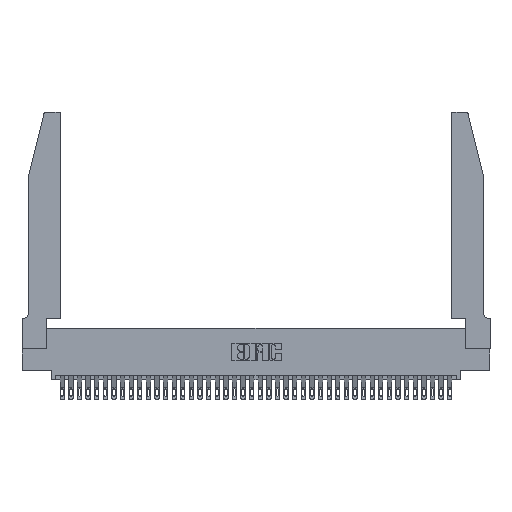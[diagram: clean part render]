
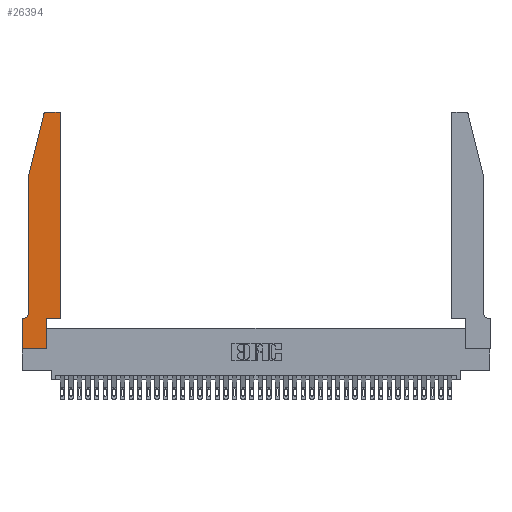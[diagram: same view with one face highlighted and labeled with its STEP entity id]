
A CAD part, top view. The second image highlights one B-rep face of the part: STEP entity #26394.
In plain terms, the highlighted planar face has unit normal (0, 0, 1).
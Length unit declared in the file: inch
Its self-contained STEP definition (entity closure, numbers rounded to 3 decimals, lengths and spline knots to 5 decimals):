
#623 = CARTESIAN_POINT ( 'NONE',  ( 0.4505, 0.35, 0.37 ) ) ;
#1113 = EDGE_CURVE ( 'NONE', #15938, #35383, #37531, .T. ) ;
#1392 = EDGE_CURVE ( 'NONE', #5503, #29788, #25211, .T. ) ;
#1678 = VERTEX_POINT ( 'NONE', #5254 ) ;
#1770 = EDGE_CURVE ( 'NONE', #29566, #25575, #26668, .T. ) ;
#1964 = CARTESIAN_POINT ( 'NONE',  ( 0.4505, 2.72, 0.37 ) ) ;
#2930 = FACE_OUTER_BOUND ( 'NONE', #30927, .T. ) ;
#2972 = EDGE_CURVE ( 'NONE', #29788, #29566, #28120, .T. ) ;
#3260 = VECTOR ( 'NONE', #28836, 39.37008 ) ;
#4266 = LINE ( 'NONE', #39532, #8136 ) ;
#4419 = VECTOR ( 'NONE', #25385, 39.37008 ) ;
#4619 = VECTOR ( 'NONE', #27135, 39.37008 ) ;
#4669 = ORIENTED_EDGE ( 'NONE', *, *, #36475, .T. ) ;
#4964 = CIRCLE ( 'NONE', #12830, 0.03 ) ;
#5254 = CARTESIAN_POINT ( 'NONE',  ( 0.4505, 0.35, 0.37 ) ) ;
#5293 = ORIENTED_EDGE ( 'NONE', *, *, #1392, .T. ) ;
#5503 = VERTEX_POINT ( 'NONE', #6472 ) ;
#6472 = CARTESIAN_POINT ( 'NONE',  ( 0.0755, 0.42, 0.37 ) ) ;
#6616 = DIRECTION ( 'NONE',  ( -1., 0., 0. ) ) ;
#7291 = CARTESIAN_POINT ( 'NONE',  ( 0.2865, 0., 0.37 ) ) ;
#7638 = LINE ( 'NONE', #13547, #30873 ) ;
#7755 = VERTEX_POINT ( 'NONE', #27853 ) ;
#7964 = CARTESIAN_POINT ( 'NONE',  ( 0.2865, 0.35, 0.37 ) ) ;
#8090 = DIRECTION ( 'NONE',  ( 1., 0., 0. ) ) ;
#8136 = VECTOR ( 'NONE', #36692, 39.37008 ) ;
#8575 = CARTESIAN_POINT ( 'NONE',  ( 0.284, 2.72, 0.37 ) ) ;
#8647 = DIRECTION ( 'NONE',  ( 0., -1., 0. ) ) ;
#8649 = ORIENTED_EDGE ( 'NONE', *, *, #12506, .T. ) ;
#8650 = CARTESIAN_POINT ( 'NONE',  ( 0., 0., 0.37 ) ) ;
#9004 = EDGE_CURVE ( 'NONE', #18876, #24777, #7638, .T. ) ;
#9060 = EDGE_CURVE ( 'NONE', #1678, #15938, #4266, .T. ) ;
#9557 = LINE ( 'NONE', #29116, #27879 ) ;
#9665 = DIRECTION ( 'NONE',  ( 0., 0., -1. ) ) ;
#10341 = ORIENTED_EDGE ( 'NONE', *, *, #37391, .T. ) ;
#10510 = ORIENTED_EDGE ( 'NONE', *, *, #31193, .T. ) ;
#10764 = CARTESIAN_POINT ( 'NONE',  ( 0., 0.35, 0.37 ) ) ;
#11015 = ORIENTED_EDGE ( 'NONE', *, *, #1770, .T. ) ;
#12506 = EDGE_CURVE ( 'NONE', #13394, #13069, #24665, .T. ) ;
#12652 = ORIENTED_EDGE ( 'NONE', *, *, #9004, .T. ) ;
#12830 = AXIS2_PLACEMENT_3D ( 'NONE', #8575, #24651, #21610 ) ;
#13069 = VERTEX_POINT ( 'NONE', #33741 ) ;
#13394 = VERTEX_POINT ( 'NONE', #38401 ) ;
#13547 = CARTESIAN_POINT ( 'NONE',  ( 0.2865, 0.35, 0.37 ) ) ;
#14224 = DIRECTION ( 'NONE',  ( -1., 0., 0. ) ) ;
#15938 = VERTEX_POINT ( 'NONE', #1964 ) ;
#17227 = DIRECTION ( 'NONE',  ( 1., 0., 0. ) ) ;
#17337 = CARTESIAN_POINT ( 'NONE',  ( 0.4205, 2.72, 0.37 ) ) ;
#18331 = ORIENTED_EDGE ( 'NONE', *, *, #2972, .T. ) ;
#18876 = VERTEX_POINT ( 'NONE', #7291 ) ;
#19086 = CARTESIAN_POINT ( 'NONE',  ( 0.0055, 0.42, 0.37 ) ) ;
#19629 = EDGE_CURVE ( 'NONE', #7755, #13394, #4964, .T. ) ;
#21147 = VECTOR ( 'NONE', #14224, 39.37008 ) ;
#21576 = DIRECTION ( 'NONE',  ( 0., -1., 0. ) ) ;
#21610 = DIRECTION ( 'NONE',  ( 1., 0., 0. ) ) ;
#22152 = CARTESIAN_POINT ( 'NONE',  ( 0.0055, 0.35, 0.37 ) ) ;
#22228 = VECTOR ( 'NONE', #8647, 39.37008 ) ;
#22506 = LINE ( 'NONE', #623, #3260 ) ;
#23856 = ORIENTED_EDGE ( 'NONE', *, *, #31564, .T. ) ;
#24651 = DIRECTION ( 'NONE',  ( 0., 0., 1. ) ) ;
#24665 = LINE ( 'NONE', #29022, #4419 ) ;
#24777 = VERTEX_POINT ( 'NONE', #7964 ) ;
#25211 = CIRCLE ( 'NONE', #33574, 0.07 ) ;
#25385 = DIRECTION ( 'NONE',  ( -0.239, -0.971, 0. ) ) ;
#25575 = VERTEX_POINT ( 'NONE', #8650 ) ;
#25917 = DIRECTION ( 'NONE',  ( 1., 0., 0. ) ) ;
#26025 = CARTESIAN_POINT ( 'NONE',  ( 0.0755, 0.35, 0.37 ) ) ;
#26394 = ADVANCED_FACE ( 'NONE', ( #2930 ), #32864, .T. ) ;
#26618 = AXIS2_PLACEMENT_3D ( 'NONE', #17337, #27053, #8090 ) ;
#26668 = LINE ( 'NONE', #27338, #22228 ) ;
#26930 = CARTESIAN_POINT ( 'NONE',  ( 0., 0.35, 0.37 ) ) ;
#27053 = DIRECTION ( 'NONE',  ( 0., 0., 1. ) ) ;
#27135 = DIRECTION ( 'NONE',  ( -1., 0., 0. ) ) ;
#27338 = CARTESIAN_POINT ( 'NONE',  ( 0., 0., 0.37 ) ) ;
#27853 = CARTESIAN_POINT ( 'NONE',  ( 0.284, 2.75, 0.37 ) ) ;
#27879 = VECTOR ( 'NONE', #25917, 39.37008 ) ;
#28120 = LINE ( 'NONE', #26025, #21147 ) ;
#28436 = VECTOR ( 'NONE', #21576, 39.37008 ) ;
#28836 = DIRECTION ( 'NONE',  ( 1., 0., 0. ) ) ;
#28933 = LINE ( 'NONE', #34242, #28436 ) ;
#29022 = CARTESIAN_POINT ( 'NONE',  ( 0.0755, 2., 0.37 ) ) ;
#29116 = CARTESIAN_POINT ( 'NONE',  ( 0., 0., 0.37 ) ) ;
#29490 = CARTESIAN_POINT ( 'NONE',  ( 0.4205, 2.75, 0.37 ) ) ;
#29566 = VERTEX_POINT ( 'NONE', #10764 ) ;
#29788 = VERTEX_POINT ( 'NONE', #22152 ) ;
#30873 = VECTOR ( 'NONE', #30973, 39.37008 ) ;
#30927 = EDGE_LOOP ( 'NONE', ( #23856, #32319, #8649, #10341, #5293, #18331, #11015, #10510, #12652, #4669, #37583, #39095 ) ) ;
#30973 = DIRECTION ( 'NONE',  ( 0., 1., 0. ) ) ;
#31193 = EDGE_CURVE ( 'NONE', #25575, #18876, #9557, .T. ) ;
#31564 = EDGE_CURVE ( 'NONE', #35383, #7755, #36206, .T. ) ;
#32319 = ORIENTED_EDGE ( 'NONE', *, *, #19629, .T. ) ;
#32864 = PLANE ( 'NONE',  #40697 ) ;
#33574 = AXIS2_PLACEMENT_3D ( 'NONE', #19086, #9665, #6616 ) ;
#33741 = CARTESIAN_POINT ( 'NONE',  ( 0.0755, 2., 0.37 ) ) ;
#34242 = CARTESIAN_POINT ( 'NONE',  ( 0.0755, 2., 0.37 ) ) ;
#35383 = VERTEX_POINT ( 'NONE', #29490 ) ;
#36168 = DIRECTION ( 'NONE',  ( 0., 0., 1. ) ) ;
#36206 = LINE ( 'NONE', #39599, #4619 ) ;
#36475 = EDGE_CURVE ( 'NONE', #24777, #1678, #22506, .T. ) ;
#36692 = DIRECTION ( 'NONE',  ( 0., 1., 0. ) ) ;
#37391 = EDGE_CURVE ( 'NONE', #13069, #5503, #28933, .T. ) ;
#37531 = CIRCLE ( 'NONE', #26618, 0.03 ) ;
#37583 = ORIENTED_EDGE ( 'NONE', *, *, #9060, .T. ) ;
#38401 = CARTESIAN_POINT ( 'NONE',  ( 0.25487, 2.72718, 0.37 ) ) ;
#39095 = ORIENTED_EDGE ( 'NONE', *, *, #1113, .T. ) ;
#39532 = CARTESIAN_POINT ( 'NONE',  ( 0.4505, 0.35, 0.37 ) ) ;
#39599 = CARTESIAN_POINT ( 'NONE',  ( 0.2605, 2.75, 0.37 ) ) ;
#40697 = AXIS2_PLACEMENT_3D ( 'NONE', #26930, #36168, #17227 ) ;
